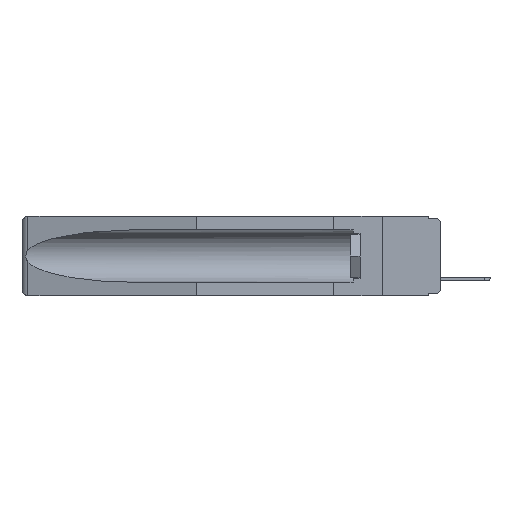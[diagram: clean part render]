
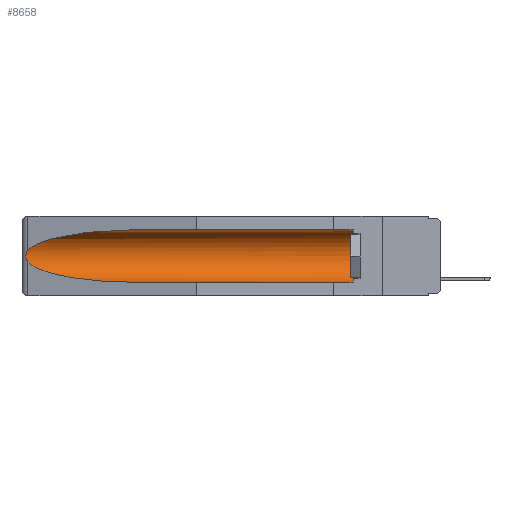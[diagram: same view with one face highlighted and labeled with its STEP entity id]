
A CAD part, left-side view. The second image highlights one B-rep face of the part: STEP entity #8658.
In plain terms, the highlighted cylindrical face has radius 2.857 mm (diameter 5.715 mm), a partial arc.
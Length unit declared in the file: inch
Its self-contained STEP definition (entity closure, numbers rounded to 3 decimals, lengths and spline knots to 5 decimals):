
#963 = LINE ( 'NONE', #21623, #11523 ) ;
#1119 = CARTESIAN_POINT ( 'NONE',  ( 0.25451, 1.48313, -0.24835 ) ) ;
#1316 = EDGE_CURVE ( 'NONE', #15595, #15577, #4902, .T. ) ;
#1451 = EDGE_LOOP ( 'NONE', ( #4844, #14108, #3047, #3768, #20931, #6597 ) ) ;
#1575 = CARTESIAN_POINT ( 'NONE',  ( 0.26597, 1.52961, -0.15275 ) ) ;
#1718 = DIRECTION ( 'NONE',  ( 0., 1., 0. ) ) ;
#1827 = VERTEX_POINT ( 'NONE', #12476 ) ;
#2207 = CARTESIAN_POINT ( 'NONE',  ( 0.155, 1.07973, -0.284 ) ) ;
#3025 =( BOUNDED_CURVE ( )  B_SPLINE_CURVE ( 3, ( #8120, #1119, #6626, #17030 ),
 .UNSPECIFIED., .F., .F. ) 
 B_SPLINE_CURVE_WITH_KNOTS ( ( 4, 4 ),
 ( 0.1948, 1.5708 ),
 .UNSPECIFIED. ) 
 CURVE ( )  GEOMETRIC_REPRESENTATION_ITEM ( )  RATIONAL_B_SPLINE_CURVE ( ( 1., 0.848, 0.848, 1. ) ) 
 REPRESENTATION_ITEM ( '' )  );
#3047 = ORIENTED_EDGE ( 'NONE', *, *, #20009, .T. ) ;
#3132 = CARTESIAN_POINT ( 'NONE',  ( 0.155, 0.126, -0.284 ) ) ;
#3251 = CYLINDRICAL_SURFACE ( 'NONE', #11786, 0.1125 ) ;
#3768 = ORIENTED_EDGE ( 'NONE', *, *, #20353, .F. ) ;
#4410 = CARTESIAN_POINT ( 'NONE',  ( 0.26537, 1.52718, -0.14972 ) ) ;
#4844 = ORIENTED_EDGE ( 'NONE', *, *, #10397, .T. ) ;
#4902 = CIRCLE ( 'NONE', #7795, 0.1125 ) ;
#4957 = DIRECTION ( 'NONE',  ( 0., -1., 0. ) ) ;
#5073 = CARTESIAN_POINT ( 'NONE',  ( 0.26655, 1.53094, -0.18657 ) ) ;
#5176 = DIRECTION ( 'NONE',  ( 0., 0., 1. ) ) ;
#6209 = CARTESIAN_POINT ( 'NONE',  ( 0.155, 1.07973, -0.059 ) ) ;
#6308 = CARTESIAN_POINT ( 'NONE',  ( 0.155, 0.126, -0.059 ) ) ;
#6536 = CARTESIAN_POINT ( 'NONE',  ( 0.2675, 1.53308, -0.16763 ) ) ;
#6597 = ORIENTED_EDGE ( 'NONE', *, *, #17763, .T. ) ;
#6625 = CARTESIAN_POINT ( 'NONE',  ( 0.26537, 1.52718, -0.14972 ) ) ;
#6626 = CARTESIAN_POINT ( 'NONE',  ( 0.21114, 1.30732, -0.284 ) ) ;
#7075 = CARTESIAN_POINT ( 'NONE',  ( 0.26537, 1.52718, -0.19328 ) ) ;
#7427 = B_SPLINE_CURVE_WITH_KNOTS ( 'NONE', 3,
 ( #17051, #1575, #13334, #8466, #6536, #22230, #13650, #5073, #16726, #11967 ),
 .UNSPECIFIED., .F., .F.,
 ( 4, 2, 2, 2, 4 ),
 ( 0., 0.00029, 0.00058, 0.00087, 0.00117 ),
 .UNSPECIFIED. ) ;
#7795 = AXIS2_PLACEMENT_3D ( 'NONE', #8571, #4957, #11866 ) ;
#8120 = CARTESIAN_POINT ( 'NONE',  ( 0.26537, 1.52718, -0.19328 ) ) ;
#8451 = DIRECTION ( 'NONE',  ( 0., 1., 0. ) ) ;
#8466 = CARTESIAN_POINT ( 'NONE',  ( 0.2673, 1.5327, -0.16383 ) ) ;
#8571 = CARTESIAN_POINT ( 'NONE',  ( 0.155, 0.126, -0.1715 ) ) ;
#8638 = VERTEX_POINT ( 'NONE', #7075 ) ;
#8658 = ADVANCED_FACE ( 'NONE', ( #20859 ), #3251, .F. ) ;
#10397 = EDGE_CURVE ( 'NONE', #1827, #14308, #20765, .T. ) ;
#11523 = VECTOR ( 'NONE', #13037, 39.37008 ) ;
#11786 = AXIS2_PLACEMENT_3D ( 'NONE', #15451, #8451, #5176 ) ;
#11844 = EDGE_CURVE ( 'NONE', #14308, #8638, #7427, .T. ) ;
#11866 = DIRECTION ( 'NONE',  ( 0., 0., 1. ) ) ;
#11967 = CARTESIAN_POINT ( 'NONE',  ( 0.26537, 1.52718, -0.19328 ) ) ;
#12476 = CARTESIAN_POINT ( 'NONE',  ( 0.155, 1.07973, -0.059 ) ) ;
#12587 = VERTEX_POINT ( 'NONE', #2207 ) ;
#12661 = CARTESIAN_POINT ( 'NONE',  ( 0.21114, 1.30732, -0.059 ) ) ;
#13037 = DIRECTION ( 'NONE',  ( 0., 1., 0. ) ) ;
#13334 = CARTESIAN_POINT ( 'NONE',  ( 0.26654, 1.53092, -0.15636 ) ) ;
#13372 = LINE ( 'NONE', #15280, #18107 ) ;
#13650 = CARTESIAN_POINT ( 'NONE',  ( 0.2673, 1.53269, -0.17917 ) ) ;
#14108 = ORIENTED_EDGE ( 'NONE', *, *, #11844, .T. ) ;
#14308 = VERTEX_POINT ( 'NONE', #6625 ) ;
#15280 = CARTESIAN_POINT ( 'NONE',  ( 0.155, -0.30754, -0.284 ) ) ;
#15451 = CARTESIAN_POINT ( 'NONE',  ( 0.155, -0.30754, -0.1715 ) ) ;
#15577 = VERTEX_POINT ( 'NONE', #6308 ) ;
#15595 = VERTEX_POINT ( 'NONE', #3132 ) ;
#16726 = CARTESIAN_POINT ( 'NONE',  ( 0.26597, 1.5296, -0.19026 ) ) ;
#17030 = CARTESIAN_POINT ( 'NONE',  ( 0.155, 1.07973, -0.284 ) ) ;
#17051 = CARTESIAN_POINT ( 'NONE',  ( 0.26537, 1.52718, -0.14972 ) ) ;
#17763 = EDGE_CURVE ( 'NONE', #15577, #1827, #963, .T. ) ;
#18107 = VECTOR ( 'NONE', #1718, 39.37008 ) ;
#20009 = EDGE_CURVE ( 'NONE', #8638, #12587, #3025, .T. ) ;
#20353 = EDGE_CURVE ( 'NONE', #15595, #12587, #13372, .T. ) ;
#20765 =( BOUNDED_CURVE ( )  B_SPLINE_CURVE ( 3, ( #6209, #12661, #21680, #4410 ),
 .UNSPECIFIED., .F., .F. ) 
 B_SPLINE_CURVE_WITH_KNOTS ( ( 4, 4 ),
 ( 4.71239, 6.08839 ),
 .UNSPECIFIED. ) 
 CURVE ( )  GEOMETRIC_REPRESENTATION_ITEM ( )  RATIONAL_B_SPLINE_CURVE ( ( 1., 0.848, 0.848, 1. ) ) 
 REPRESENTATION_ITEM ( '' )  );
#20859 = FACE_OUTER_BOUND ( 'NONE', #1451, .T. ) ;
#20931 = ORIENTED_EDGE ( 'NONE', *, *, #1316, .T. ) ;
#21623 = CARTESIAN_POINT ( 'NONE',  ( 0.155, -0.30754, -0.059 ) ) ;
#21680 = CARTESIAN_POINT ( 'NONE',  ( 0.25451, 1.48313, -0.09465 ) ) ;
#22230 = CARTESIAN_POINT ( 'NONE',  ( 0.2675, 1.53308, -0.17534 ) ) ;
